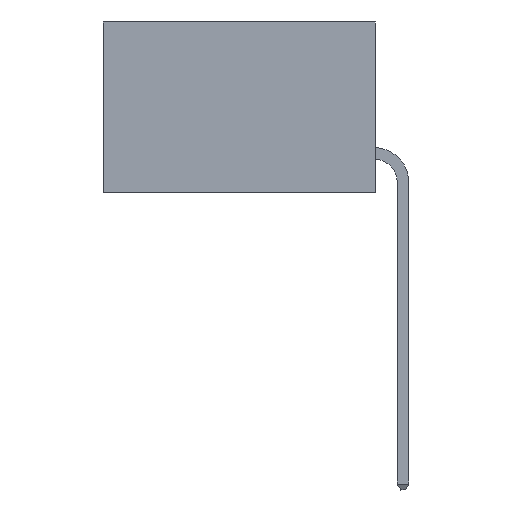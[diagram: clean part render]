
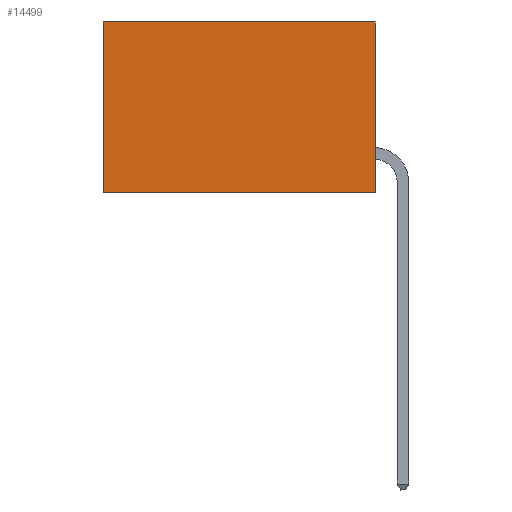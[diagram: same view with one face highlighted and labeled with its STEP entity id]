
A CAD part, left-side view. The second image highlights one B-rep face of the part: STEP entity #14499.
In plain terms, the highlighted planar face has unit normal (-1, 0, 0).
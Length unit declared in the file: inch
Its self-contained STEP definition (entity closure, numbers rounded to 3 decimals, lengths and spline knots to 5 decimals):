
#4 = LINE ( 'NONE', #15215, #22307 ) ;
#350 = DIRECTION ( 'NONE',  ( 0., 0., -1. ) ) ;
#574 = VERTEX_POINT ( 'NONE', #9688 ) ;
#967 = FACE_OUTER_BOUND ( 'NONE', #24506, .T. ) ;
#2765 = VECTOR ( 'NONE', #9116, 39.37008 ) ;
#4102 = EDGE_CURVE ( 'NONE', #26742, #21531, #25498, .T. ) ;
#4149 = EDGE_CURVE ( 'NONE', #574, #26742, #14771, .T. ) ;
#4441 = PLANE ( 'NONE',  #18641 ) ;
#4536 = CARTESIAN_POINT ( 'NONE',  ( 0.277, 0.59, -0.37 ) ) ;
#6031 = LINE ( 'NONE', #8135, #22632 ) ;
#6258 = CARTESIAN_POINT ( 'NONE',  ( 0.277, 0.59, 0. ) ) ;
#6582 = DIRECTION ( 'NONE',  ( 0., 0., -1. ) ) ;
#7791 = VERTEX_POINT ( 'NONE', #21752 ) ;
#8135 = CARTESIAN_POINT ( 'NONE',  ( 0.277, 0., -0.37 ) ) ;
#9116 = DIRECTION ( 'NONE',  ( 0., 1., 0. ) ) ;
#9268 = CARTESIAN_POINT ( 'NONE',  ( 0.277, 0., 0. ) ) ;
#9688 = CARTESIAN_POINT ( 'NONE',  ( 0.277, 0., 0. ) ) ;
#9929 = DIRECTION ( 'NONE',  ( 0., 0., -1. ) ) ;
#10254 = ORIENTED_EDGE ( 'NONE', *, *, #12058, .F. ) ;
#10425 = CARTESIAN_POINT ( 'NONE',  ( 0.277, 0.59, -0.37 ) ) ;
#11600 = EDGE_CURVE ( 'NONE', #574, #7791, #4, .T. ) ;
#12058 = EDGE_CURVE ( 'NONE', #7791, #21531, #6031, .T. ) ;
#13513 = ORIENTED_EDGE ( 'NONE', *, *, #4149, .T. ) ;
#14499 = ADVANCED_FACE ( 'NONE', ( #967 ), #4441, .F. ) ;
#14771 = LINE ( 'NONE', #9268, #2765 ) ;
#15215 = CARTESIAN_POINT ( 'NONE',  ( 0.277, 0., -0.37 ) ) ;
#17131 = CARTESIAN_POINT ( 'NONE',  ( 0.277, 0., -0.37 ) ) ;
#18641 = AXIS2_PLACEMENT_3D ( 'NONE', #17131, #19141, #6582 ) ;
#19141 = DIRECTION ( 'NONE',  ( 1., 0., 0. ) ) ;
#19679 = ORIENTED_EDGE ( 'NONE', *, *, #4102, .T. ) ;
#20217 = VECTOR ( 'NONE', #9929, 39.37008 ) ;
#20648 = DIRECTION ( 'NONE',  ( 0., 1., 0. ) ) ;
#20923 = ORIENTED_EDGE ( 'NONE', *, *, #11600, .F. ) ;
#21531 = VERTEX_POINT ( 'NONE', #4536 ) ;
#21752 = CARTESIAN_POINT ( 'NONE',  ( 0.277, 0., -0.37 ) ) ;
#22307 = VECTOR ( 'NONE', #350, 39.37008 ) ;
#22632 = VECTOR ( 'NONE', #20648, 39.37008 ) ;
#24506 = EDGE_LOOP ( 'NONE', ( #19679, #10254, #20923, #13513 ) ) ;
#25498 = LINE ( 'NONE', #10425, #20217 ) ;
#26742 = VERTEX_POINT ( 'NONE', #6258 ) ;
